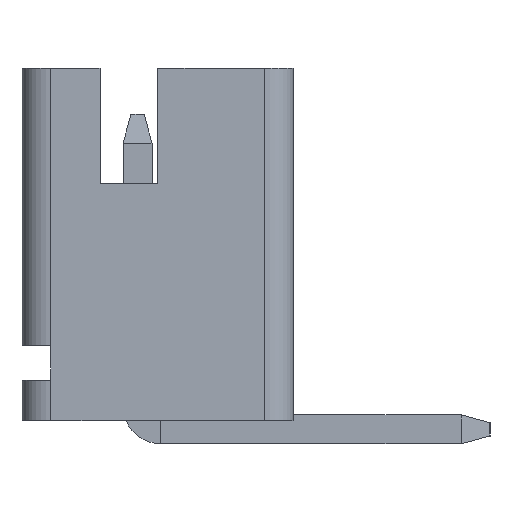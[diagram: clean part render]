
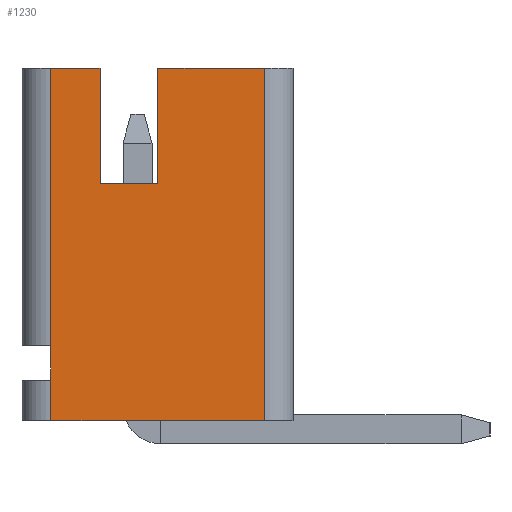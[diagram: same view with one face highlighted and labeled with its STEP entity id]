
A CAD part, left-side view. The second image highlights one B-rep face of the part: STEP entity #1230.
In plain terms, the highlighted planar face has unit normal (-1, 0, 0).
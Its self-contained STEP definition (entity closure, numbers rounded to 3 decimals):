
#167 = EDGE_CURVE ( 'NONE', #729, #3545, #709, .T. ) ;
#168 = EDGE_CURVE ( 'NONE', #4441, #562, #2338, .T. ) ;
#341 = DIRECTION ( 'NONE',  ( 0., 0., -1. ) ) ;
#385 = CARTESIAN_POINT ( 'NONE',  ( -2., 0.65, 4.1 ) ) ;
#400 = VERTEX_POINT ( 'NONE', #2140 ) ;
#499 = ORIENTED_EDGE ( 'NONE', *, *, #167, .T. ) ;
#562 = VERTEX_POINT ( 'NONE', #385 ) ;
#613 = ORIENTED_EDGE ( 'NONE', *, *, #2525, .T. ) ;
#664 = VECTOR ( 'NONE', #4502, 1000. ) ;
#705 = PLANE ( 'NONE',  #2837 ) ;
#709 = LINE ( 'NONE', #3503, #4391 ) ;
#729 = VERTEX_POINT ( 'NONE', #2601 ) ;
#837 = CARTESIAN_POINT ( 'NONE',  ( -2., 0.65, 6.1 ) ) ;
#965 = CARTESIAN_POINT ( 'NONE',  ( -2., -2.2, 0. ) ) ;
#969 = CARTESIAN_POINT ( 'NONE',  ( -2., 1.5, 0. ) ) ;
#1065 = VERTEX_POINT ( 'NONE', #4062 ) ;
#1230 = ADVANCED_FACE ( 'NONE', ( #1514 ), #705, .T. ) ;
#1247 = LINE ( 'NONE', #3599, #4741 ) ;
#1257 = CARTESIAN_POINT ( 'NONE',  ( -2., 1.5, 1.3 ) ) ;
#1325 = CARTESIAN_POINT ( 'NONE',  ( -2., 1.5, 0. ) ) ;
#1514 = FACE_OUTER_BOUND ( 'NONE', #4258, .T. ) ;
#1541 = LINE ( 'NONE', #3500, #1663 ) ;
#1563 = DIRECTION ( 'NONE',  ( 0., 0., -1. ) ) ;
#1663 = VECTOR ( 'NONE', #341, 1000. ) ;
#1727 = CARTESIAN_POINT ( 'NONE',  ( -2., 2., 0. ) ) ;
#1801 = DIRECTION ( 'NONE',  ( 0., 0., 1. ) ) ;
#1900 = VECTOR ( 'NONE', #3551, 1000. ) ;
#1954 = LINE ( 'NONE', #2356, #4599 ) ;
#2036 = EDGE_CURVE ( 'NONE', #3103, #400, #4123, .T. ) ;
#2097 = ORIENTED_EDGE ( 'NONE', *, *, #3987, .T. ) ;
#2140 = CARTESIAN_POINT ( 'NONE',  ( -2., -0.35, 6.1 ) ) ;
#2280 = DIRECTION ( 'NONE',  ( 0., 0., -1. ) ) ;
#2295 = VERTEX_POINT ( 'NONE', #2849 ) ;
#2298 = ORIENTED_EDGE ( 'NONE', *, *, #2472, .T. ) ;
#2318 = VECTOR ( 'NONE', #2339, 1000. ) ;
#2338 = LINE ( 'NONE', #3863, #1900 ) ;
#2339 = DIRECTION ( 'NONE',  ( 0., 0., 1. ) ) ;
#2356 = CARTESIAN_POINT ( 'NONE',  ( -2., 2., 6.1 ) ) ;
#2472 = EDGE_CURVE ( 'NONE', #2295, #3103, #4089, .T. ) ;
#2525 = EDGE_CURVE ( 'NONE', #1065, #5122, #3391, .T. ) ;
#2544 = VERTEX_POINT ( 'NONE', #4972 ) ;
#2601 = CARTESIAN_POINT ( 'NONE',  ( -2., 1.5, 6.1 ) ) ;
#2618 = CARTESIAN_POINT ( 'NONE',  ( -2., -0.35, 6.1 ) ) ;
#2641 = EDGE_CURVE ( 'NONE', #400, #4441, #1541, .T. ) ;
#2690 = DIRECTION ( 'NONE',  ( -1., 0., 0. ) ) ;
#2755 = EDGE_CURVE ( 'NONE', #3545, #1065, #1247, .T. ) ;
#2837 = AXIS2_PLACEMENT_3D ( 'NONE', #4970, #2690, #3473 ) ;
#2849 = CARTESIAN_POINT ( 'NONE',  ( -2., -2.2, 0. ) ) ;
#2931 = DIRECTION ( 'NONE',  ( 0., 1., 0. ) ) ;
#2991 = ORIENTED_EDGE ( 'NONE', *, *, #3227, .T. ) ;
#3023 = ORIENTED_EDGE ( 'NONE', *, *, #3730, .T. ) ;
#3103 = VERTEX_POINT ( 'NONE', #3881 ) ;
#3227 = EDGE_CURVE ( 'NONE', #2544, #729, #1954, .T. ) ;
#3369 = DIRECTION ( 'NONE',  ( 0., -1., 0. ) ) ;
#3391 = LINE ( 'NONE', #1325, #664 ) ;
#3410 = VECTOR ( 'NONE', #2931, 1000. ) ;
#3448 = ORIENTED_EDGE ( 'NONE', *, *, #2641, .T. ) ;
#3473 = DIRECTION ( 'NONE',  ( 0., -1., 0. ) ) ;
#3500 = CARTESIAN_POINT ( 'NONE',  ( -2., -0.35, 6.1 ) ) ;
#3503 = CARTESIAN_POINT ( 'NONE',  ( -2., 1.5, 0. ) ) ;
#3543 = DIRECTION ( 'NONE',  ( 0., 1., 0. ) ) ;
#3545 = VERTEX_POINT ( 'NONE', #1257 ) ;
#3551 = DIRECTION ( 'NONE',  ( 0., 1., 0. ) ) ;
#3599 = CARTESIAN_POINT ( 'NONE',  ( -2., 1.5, 1.3 ) ) ;
#3664 = VECTOR ( 'NONE', #1801, 1000. ) ;
#3727 = ORIENTED_EDGE ( 'NONE', *, *, #168, .T. ) ;
#3730 = EDGE_CURVE ( 'NONE', #5122, #2295, #4480, .T. ) ;
#3863 = CARTESIAN_POINT ( 'NONE',  ( -2., 0.65, 4.1 ) ) ;
#3881 = CARTESIAN_POINT ( 'NONE',  ( -2., -2.2, 6.1 ) ) ;
#3987 = EDGE_CURVE ( 'NONE', #562, #2544, #4818, .T. ) ;
#4062 = CARTESIAN_POINT ( 'NONE',  ( -2., 1.5, 0.7 ) ) ;
#4089 = LINE ( 'NONE', #965, #3664 ) ;
#4123 = LINE ( 'NONE', #2618, #3410 ) ;
#4159 = ORIENTED_EDGE ( 'NONE', *, *, #2036, .T. ) ;
#4258 = EDGE_LOOP ( 'NONE', ( #3023, #2298, #4159, #3448, #3727, #2097, #2991, #499, #4259, #613 ) ) ;
#4259 = ORIENTED_EDGE ( 'NONE', *, *, #2755, .T. ) ;
#4295 = CARTESIAN_POINT ( 'NONE',  ( -2., -0.35, 4.1 ) ) ;
#4391 = VECTOR ( 'NONE', #2280, 1000. ) ;
#4441 = VERTEX_POINT ( 'NONE', #4295 ) ;
#4480 = LINE ( 'NONE', #1727, #4959 ) ;
#4502 = DIRECTION ( 'NONE',  ( 0., 0., -1. ) ) ;
#4599 = VECTOR ( 'NONE', #3543, 1000. ) ;
#4741 = VECTOR ( 'NONE', #1563, 1000. ) ;
#4818 = LINE ( 'NONE', #837, #2318 ) ;
#4959 = VECTOR ( 'NONE', #3369, 1000. ) ;
#4970 = CARTESIAN_POINT ( 'NONE',  ( -2., 0., 0. ) ) ;
#4972 = CARTESIAN_POINT ( 'NONE',  ( -2., 0.65, 6.1 ) ) ;
#5122 = VERTEX_POINT ( 'NONE', #969 ) ;
